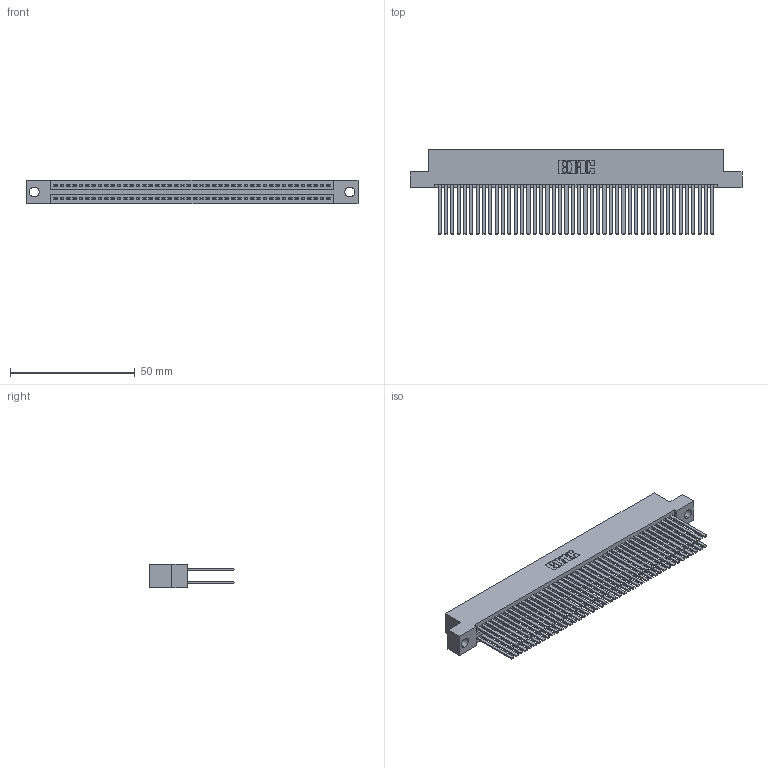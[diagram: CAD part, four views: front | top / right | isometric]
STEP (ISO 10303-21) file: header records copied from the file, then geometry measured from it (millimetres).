
FILE_DESCRIPTION (( 'STEP AP203' ), '1' );
FILE_NAME ('345-088-544-204.STEP', '2021-05-20T14:15:06', ( '' ), ( '' ), 'SwSTEP 2.0', 'SolidWorks 2020', '' );
FILE_SCHEMA (( 'CONFIG_CONTROL_DESIGN' ));
Length unit declared in the file: inch
Products named in the file (3): 345-292-001_345-293-144; 345-088-544-204; 345 Part_Flush Mounting Lugs - 0.156 Dia-TI
Assembly tree (89 placements, depth 2):
  345-088-544-204
    345 Part_Flush Mounting Lugs - 0.156 Dia-TI
    345-292-001_345-293-144  x88
Bounding box: 132.97 x 33.96 x 9.4 mm (x, y, z)
Volume: 14063 mm3; surface area: 24293.3 mm2
Topology: 89 solids, 89 shells, 4012 faces, 11905 edges, 7818 vertices
Faces by surface type: plane 2646, cylinder 1366
Entity records: 34489 total; most frequent: CARTESIAN_POINT 5782, ORIENTED_EDGE 5714, DIRECTION 5093, EDGE_CURVE 2857, VECTOR 2553, LINE 2553, VERTEX_POINT 1902, AXIS2_PLACEMENT_3D 1270
